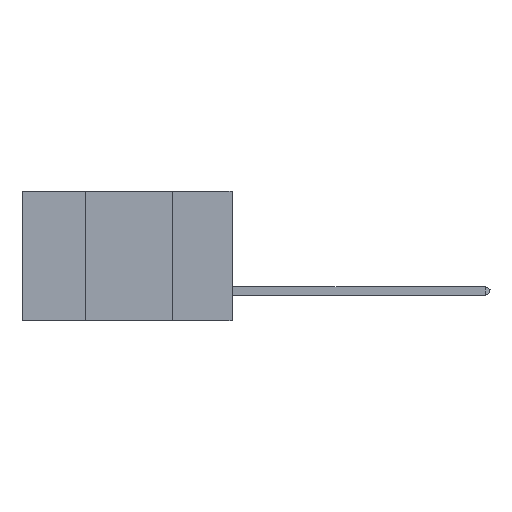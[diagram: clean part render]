
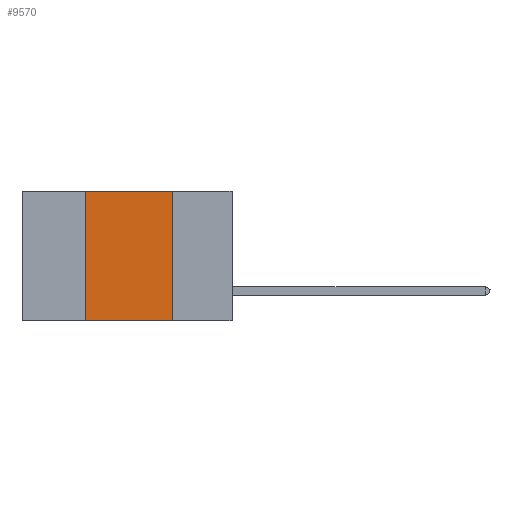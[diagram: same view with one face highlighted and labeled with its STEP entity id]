
A CAD part, left-side view. The second image highlights one B-rep face of the part: STEP entity #9570.
In plain terms, the highlighted planar face has unit normal (-1, 0, 0).
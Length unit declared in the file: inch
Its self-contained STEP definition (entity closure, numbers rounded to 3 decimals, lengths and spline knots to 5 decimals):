
#110 = DIRECTION ( 'NONE',  ( 0., 0., -1. ) ) ;
#333 = VERTEX_POINT ( 'NONE', #16990 ) ;
#1467 = CARTESIAN_POINT ( 'NONE',  ( 0., 0.42, -0.37 ) ) ;
#1667 = VECTOR ( 'NONE', #20141, 39.37008 ) ;
#1891 = ORIENTED_EDGE ( 'NONE', *, *, #19232, .F. ) ;
#2696 = AXIS2_PLACEMENT_3D ( 'NONE', #7885, #21921, #15055 ) ;
#3893 = ORIENTED_EDGE ( 'NONE', *, *, #5050, .T. ) ;
#4962 = EDGE_CURVE ( 'NONE', #21883, #14936, #12734, .T. ) ;
#5050 = EDGE_CURVE ( 'NONE', #21883, #333, #15227, .T. ) ;
#5484 = EDGE_LOOP ( 'NONE', ( #10226, #1891, #22137, #3893 ) ) ;
#7807 = CARTESIAN_POINT ( 'NONE',  ( 0., 0.6, 0. ) ) ;
#7885 = CARTESIAN_POINT ( 'NONE',  ( 0., 0.6, 0. ) ) ;
#8388 = DIRECTION ( 'NONE',  ( 0., -1., 0. ) ) ;
#9570 = ADVANCED_FACE ( 'NONE', ( #12929 ), #18439, .F. ) ;
#9914 = DIRECTION ( 'NONE',  ( 0., 0., 1. ) ) ;
#10226 = ORIENTED_EDGE ( 'NONE', *, *, #22313, .F. ) ;
#10494 = LINE ( 'NONE', #19342, #21245 ) ;
#10504 = VECTOR ( 'NONE', #8388, 39.37008 ) ;
#11042 = VECTOR ( 'NONE', #9914, 39.37008 ) ;
#12734 = LINE ( 'NONE', #19845, #11042 ) ;
#12929 = FACE_OUTER_BOUND ( 'NONE', #5484, .T. ) ;
#14936 = VERTEX_POINT ( 'NONE', #20839 ) ;
#15055 = DIRECTION ( 'NONE',  ( 0., 0., -1. ) ) ;
#15227 = LINE ( 'NONE', #21480, #10504 ) ;
#15720 = LINE ( 'NONE', #7807, #1667 ) ;
#16990 = CARTESIAN_POINT ( 'NONE',  ( 0., 0.17, -0.37 ) ) ;
#17962 = CARTESIAN_POINT ( 'NONE',  ( 0., 0.17, 0. ) ) ;
#18439 = PLANE ( 'NONE',  #2696 ) ;
#18757 = VERTEX_POINT ( 'NONE', #17962 ) ;
#19232 = EDGE_CURVE ( 'NONE', #14936, #18757, #15720, .T. ) ;
#19342 = CARTESIAN_POINT ( 'NONE',  ( 0., 0.17, 0. ) ) ;
#19845 = CARTESIAN_POINT ( 'NONE',  ( 0., 0.42, 0. ) ) ;
#20141 = DIRECTION ( 'NONE',  ( 0., -1., 0. ) ) ;
#20839 = CARTESIAN_POINT ( 'NONE',  ( 0., 0.42, 0. ) ) ;
#21245 = VECTOR ( 'NONE', #110, 39.37008 ) ;
#21480 = CARTESIAN_POINT ( 'NONE',  ( 0., 0.6, -0.37 ) ) ;
#21883 = VERTEX_POINT ( 'NONE', #1467 ) ;
#21921 = DIRECTION ( 'NONE',  ( 1., 0., 0. ) ) ;
#22137 = ORIENTED_EDGE ( 'NONE', *, *, #4962, .F. ) ;
#22313 = EDGE_CURVE ( 'NONE', #18757, #333, #10494, .T. ) ;
